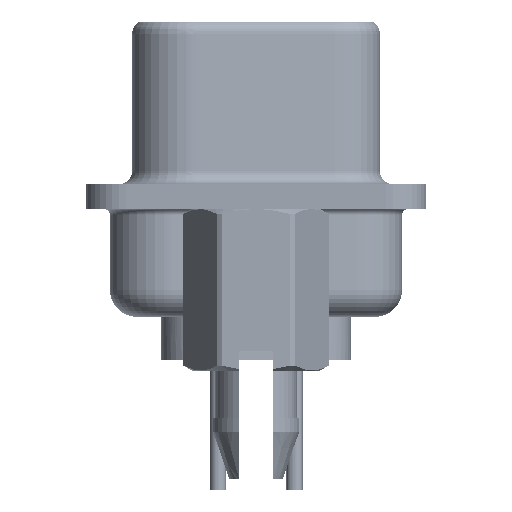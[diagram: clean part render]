
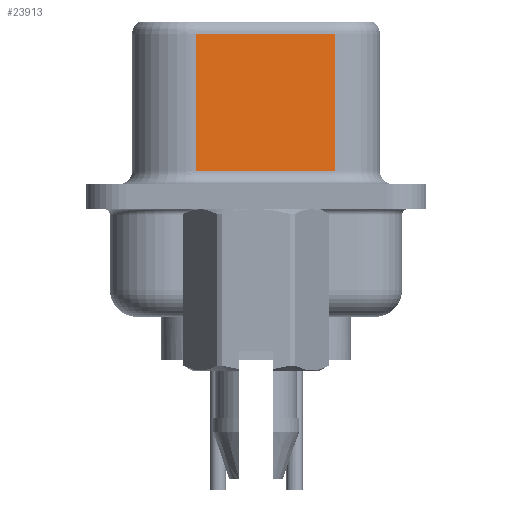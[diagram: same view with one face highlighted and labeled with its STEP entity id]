
A CAD part, left-side view. The second image highlights one B-rep face of the part: STEP entity #23913.
In plain terms, the highlighted planar face has unit normal (-0.985, -0.174, 0).
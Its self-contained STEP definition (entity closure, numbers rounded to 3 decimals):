
#1762 = DIRECTION ( 'NONE',  ( 0., 0., -1. ) ) ;
#2151 = EDGE_CURVE ( 'NONE', #29295, #11616, #21500, .T. ) ;
#2743 = EDGE_LOOP ( 'NONE', ( #16475, #6996, #28164, #3959 ) ) ;
#2819 = VECTOR ( 'NONE', #1762, 1000. ) ;
#3959 = ORIENTED_EDGE ( 'NONE', *, *, #12254, .T. ) ;
#5272 = EDGE_CURVE ( 'NONE', #11616, #16980, #11931, .T. ) ;
#6102 = LINE ( 'NONE', #27665, #2819 ) ;
#6843 = VECTOR ( 'NONE', #19698, 1000. ) ;
#6996 = ORIENTED_EDGE ( 'NONE', *, *, #2151, .T. ) ;
#7603 = VECTOR ( 'NONE', #21345, 1000. ) ;
#8546 = EDGE_CURVE ( 'NONE', #29295, #28956, #6102, .T. ) ;
#10212 = CARTESIAN_POINT ( 'NONE',  ( 3.67, 2.233, 6.52 ) ) ;
#11616 = VERTEX_POINT ( 'NONE', #25021 ) ;
#11931 = LINE ( 'NONE', #10212, #6843 ) ;
#12254 = EDGE_CURVE ( 'NONE', #16980, #28956, #21930, .T. ) ;
#12322 = CARTESIAN_POINT ( 'NONE',  ( 4.58, -2.927, 6.52 ) ) ;
#12940 = DIRECTION ( 'NONE',  ( -0.174, 0.985, 0. ) ) ;
#14131 = VECTOR ( 'NONE', #14492, 1000. ) ;
#14492 = DIRECTION ( 'NONE',  ( 0.174, -0.985, 0. ) ) ;
#15284 = DIRECTION ( 'NONE',  ( 0.985, 0.174, 0. ) ) ;
#16475 = ORIENTED_EDGE ( 'NONE', *, *, #8546, .F. ) ;
#16980 = VERTEX_POINT ( 'NONE', #30046 ) ;
#19698 = DIRECTION ( 'NONE',  ( 0., 0., -1. ) ) ;
#20834 = CARTESIAN_POINT ( 'NONE',  ( 4.58, -2.927, 0.95 ) ) ;
#21345 = DIRECTION ( 'NONE',  ( -0.174, 0.985, 0. ) ) ;
#21500 = LINE ( 'NONE', #30323, #7603 ) ;
#21930 = LINE ( 'NONE', #28615, #14131 ) ;
#22991 = CARTESIAN_POINT ( 'NONE',  ( 4.58, -2.927, 6.02 ) ) ;
#23913 = ADVANCED_FACE ( 'NONE', ( #29224 ), #26765, .F. ) ;
#25021 = CARTESIAN_POINT ( 'NONE',  ( 3.67, 2.233, 6.02 ) ) ;
#26443 = AXIS2_PLACEMENT_3D ( 'NONE', #12322, #15284, #12940 ) ;
#26765 = PLANE ( 'NONE',  #26443 ) ;
#27665 = CARTESIAN_POINT ( 'NONE',  ( 4.58, -2.927, 6.52 ) ) ;
#28164 = ORIENTED_EDGE ( 'NONE', *, *, #5272, .T. ) ;
#28615 = CARTESIAN_POINT ( 'NONE',  ( 4.58, -2.927, 0.95 ) ) ;
#28956 = VERTEX_POINT ( 'NONE', #20834 ) ;
#29224 = FACE_OUTER_BOUND ( 'NONE', #2743, .T. ) ;
#29295 = VERTEX_POINT ( 'NONE', #22991 ) ;
#30046 = CARTESIAN_POINT ( 'NONE',  ( 3.67, 2.233, 0.95 ) ) ;
#30323 = CARTESIAN_POINT ( 'NONE',  ( 4.58, -2.927, 6.02 ) ) ;
